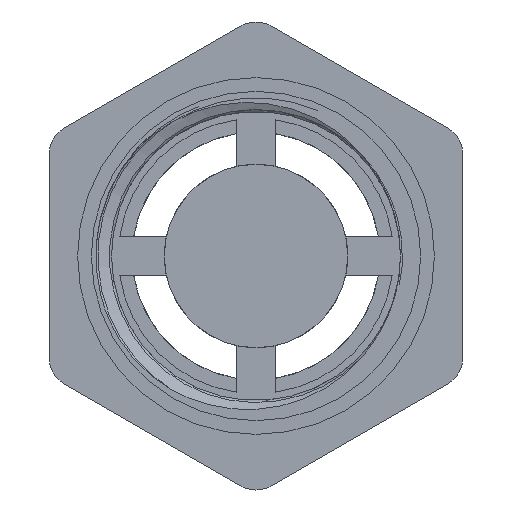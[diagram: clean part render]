
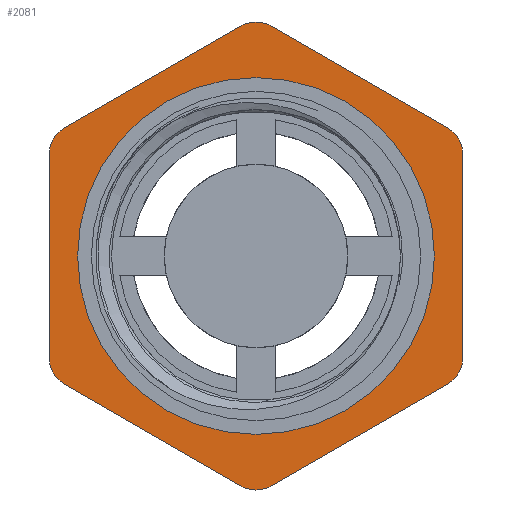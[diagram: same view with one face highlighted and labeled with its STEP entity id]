
A CAD part, front view. The second image highlights one B-rep face of the part: STEP entity #2081.
In plain terms, the highlighted planar face has unit normal (0, -1, 0).
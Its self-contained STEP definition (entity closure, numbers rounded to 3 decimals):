
#35=FACE_BOUND('',#281,.T.);
#69=PLANE('',#2300);
#168=FACE_OUTER_BOUND('',#280,.T.);
#280=EDGE_LOOP('',(#1722,#1723,#1724,#1725,#1726,#1727,#1728,#1729,#1730,
#1731,#1732,#1733));
#281=EDGE_LOOP('',(#1734));
#380=CIRCLE('',#2267,2.);
#388=CIRCLE('',#2280,2.);
#389=CIRCLE('',#2282,2.);
#390=CIRCLE('',#2285,2.);
#391=CIRCLE('',#2287,2.);
#392=CIRCLE('',#2290,2.);
#395=CIRCLE('',#2297,11.672);
#560=LINE('',#3973,#694);
#611=LINE('',#4311,#745);
#612=LINE('',#4313,#746);
#615=LINE('',#4328,#749);
#616=LINE('',#4329,#750);
#617=LINE('',#4330,#751);
#694=VECTOR('',#2543,10.);
#745=VECTOR('',#2776,10.);
#746=VECTOR('',#2779,10.);
#749=VECTOR('',#2798,10.);
#750=VECTOR('',#2799,10.);
#751=VECTOR('',#2800,10.);
#896=VERTEX_POINT('',#3970);
#897=VERTEX_POINT('',#3972);
#943=VERTEX_POINT('',#4261);
#947=VERTEX_POINT('',#4279);
#948=VERTEX_POINT('',#4280);
#949=VERTEX_POINT('',#4285);
#950=VERTEX_POINT('',#4286);
#951=VERTEX_POINT('',#4293);
#952=VERTEX_POINT('',#4294);
#953=VERTEX_POINT('',#4299);
#954=VERTEX_POINT('',#4300);
#955=VERTEX_POINT('',#4307);
#958=VERTEX_POINT('',#4321);
#1139=EDGE_CURVE('',#897,#896,#560,.T.);
#1224=EDGE_CURVE('',#897,#943,#380,.T.);
#1233=EDGE_CURVE('',#947,#948,#388,.T.);
#1236=EDGE_CURVE('',#949,#950,#389,.T.);
#1240=EDGE_CURVE('',#951,#952,#390,.T.);
#1243=EDGE_CURVE('',#953,#954,#391,.T.);
#1247=EDGE_CURVE('',#955,#896,#392,.T.);
#1249=EDGE_CURVE('',#947,#952,#611,.T.);
#1250=EDGE_CURVE('',#951,#943,#612,.T.);
#1254=EDGE_CURVE('',#958,#958,#395,.T.);
#1257=EDGE_CURVE('',#955,#954,#615,.T.);
#1258=EDGE_CURVE('',#953,#950,#616,.T.);
#1259=EDGE_CURVE('',#949,#948,#617,.T.);
#1722=ORIENTED_EDGE('',*,*,#1233,.F.);
#1723=ORIENTED_EDGE('',*,*,#1249,.T.);
#1724=ORIENTED_EDGE('',*,*,#1240,.F.);
#1725=ORIENTED_EDGE('',*,*,#1250,.T.);
#1726=ORIENTED_EDGE('',*,*,#1224,.F.);
#1727=ORIENTED_EDGE('',*,*,#1139,.T.);
#1728=ORIENTED_EDGE('',*,*,#1247,.F.);
#1729=ORIENTED_EDGE('',*,*,#1257,.T.);
#1730=ORIENTED_EDGE('',*,*,#1243,.F.);
#1731=ORIENTED_EDGE('',*,*,#1258,.T.);
#1732=ORIENTED_EDGE('',*,*,#1236,.F.);
#1733=ORIENTED_EDGE('',*,*,#1259,.T.);
#1734=ORIENTED_EDGE('',*,*,#1254,.T.);
#2081=ADVANCED_FACE('',(#168,#35),#69,.T.);
#2267=AXIS2_PLACEMENT_3D('',#4262,#2714,#2715);
#2280=AXIS2_PLACEMENT_3D('',#4281,#2741,#2742);
#2282=AXIS2_PLACEMENT_3D('',#4287,#2747,#2748);
#2285=AXIS2_PLACEMENT_3D('',#4295,#2756,#2757);
#2287=AXIS2_PLACEMENT_3D('',#4301,#2762,#2763);
#2290=AXIS2_PLACEMENT_3D('',#4308,#2771,#2772);
#2297=AXIS2_PLACEMENT_3D('',#4322,#2789,#2790);
#2300=AXIS2_PLACEMENT_3D('',#4327,#2796,#2797);
#2543=DIRECTION('',(0.,0.,1.));
#2714=DIRECTION('center_axis',(0.,1.,0.));
#2715=DIRECTION('ref_axis',(0.866,0.,-0.5));
#2741=DIRECTION('center_axis',(0.,1.,0.));
#2742=DIRECTION('ref_axis',(-0.866,0.,-0.5));
#2747=DIRECTION('center_axis',(0.,1.,0.));
#2748=DIRECTION('ref_axis',(-0.866,0.,0.5));
#2756=DIRECTION('center_axis',(0.,1.,0.));
#2757=DIRECTION('ref_axis',(0.,0.,-1.));
#2762=DIRECTION('center_axis',(0.,1.,0.));
#2763=DIRECTION('ref_axis',(0.,0.,1.));
#2771=DIRECTION('center_axis',(0.,1.,0.));
#2772=DIRECTION('ref_axis',(0.866,0.,0.5));
#2776=DIRECTION('',(0.866,0.,-0.5));
#2779=DIRECTION('',(0.866,0.,0.5));
#2789=DIRECTION('center_axis',(0.,1.,0.));
#2790=DIRECTION('ref_axis',(-1.,0.,0.));
#2796=DIRECTION('center_axis',(0.,-1.,0.));
#2797=DIRECTION('ref_axis',(0.,0.,-1.));
#2798=DIRECTION('',(-0.866,0.,0.5));
#2799=DIRECTION('',(-0.866,0.,-0.5));
#2800=DIRECTION('',(0.,0.,-1.));
#3970=CARTESIAN_POINT('',(13.524,-25.4,6.653));
#3972=CARTESIAN_POINT('',(13.524,-25.4,-6.653));
#3973=CARTESIAN_POINT('',(13.524,-25.4,-7.808));
#4261=CARTESIAN_POINT('',(12.524,-25.4,-8.385));
#4262=CARTESIAN_POINT('Origin',(11.524,-25.4,-6.653));
#4279=CARTESIAN_POINT('',(-12.524,-25.4,-8.385));
#4280=CARTESIAN_POINT('',(-13.524,-25.4,-6.653));
#4281=CARTESIAN_POINT('Origin',(-11.524,-25.4,-6.653));
#4285=CARTESIAN_POINT('',(-13.524,-25.4,6.653));
#4286=CARTESIAN_POINT('',(-12.524,-25.4,8.385));
#4287=CARTESIAN_POINT('Origin',(-11.524,-25.4,6.653));
#4293=CARTESIAN_POINT('',(1.,-25.4,-15.038));
#4294=CARTESIAN_POINT('',(-1.,-25.4,-15.038));
#4295=CARTESIAN_POINT('Origin',(0.,-25.4,-13.306));
#4299=CARTESIAN_POINT('',(-1.,-25.4,15.038));
#4300=CARTESIAN_POINT('',(1.,-25.4,15.038));
#4301=CARTESIAN_POINT('Origin',(0.,-25.4,13.306));
#4307=CARTESIAN_POINT('',(12.524,-25.4,8.385));
#4308=CARTESIAN_POINT('Origin',(11.524,-25.4,6.653));
#4311=CARTESIAN_POINT('',(-13.524,-25.4,-7.808));
#4313=CARTESIAN_POINT('',(0.,-25.4,-15.616));
#4321=CARTESIAN_POINT('',(11.672,-25.4,0.));
#4322=CARTESIAN_POINT('Origin',(0.,-25.4,0.));
#4327=CARTESIAN_POINT('Origin',(0.,-25.4,0.));
#4328=CARTESIAN_POINT('',(13.524,-25.4,7.808));
#4329=CARTESIAN_POINT('',(0.,-25.4,15.616));
#4330=CARTESIAN_POINT('',(-13.524,-25.4,7.808));
